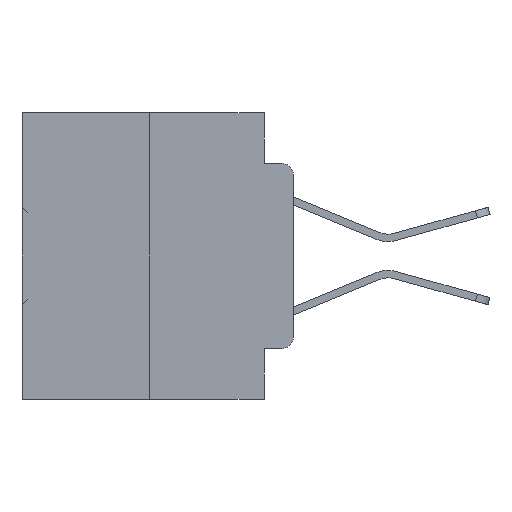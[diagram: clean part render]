
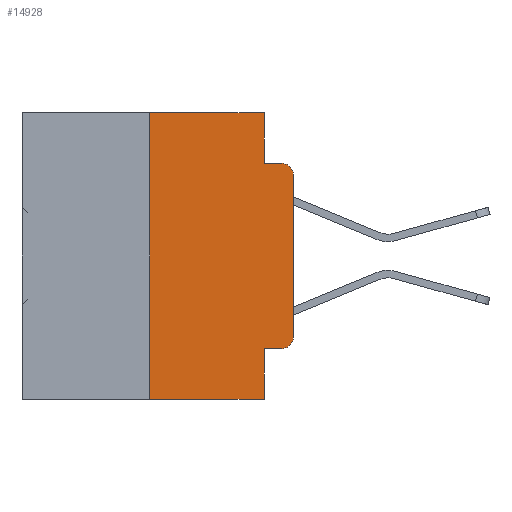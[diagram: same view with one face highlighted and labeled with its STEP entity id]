
A CAD part, left-side view. The second image highlights one B-rep face of the part: STEP entity #14928.
In plain terms, the highlighted planar face has unit normal (-1, 0, 0).
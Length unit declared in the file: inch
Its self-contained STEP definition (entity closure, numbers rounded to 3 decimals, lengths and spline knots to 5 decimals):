
#336 = AXIS2_PLACEMENT_3D ( 'NONE', #9981, #27452, #23867 ) ;
#346 = CARTESIAN_POINT ( 'NONE',  ( 0., 0.25, -0.5 ) ) ;
#2076 = LINE ( 'NONE', #24842, #9273 ) ;
#2469 = CARTESIAN_POINT ( 'NONE',  ( 0., 0.473, -0.5 ) ) ;
#2613 = VERTEX_POINT ( 'NONE', #22245 ) ;
#2767 = FACE_OUTER_BOUND ( 'NONE', #27448, .T. ) ;
#3425 = VERTEX_POINT ( 'NONE', #19836 ) ;
#4374 = CARTESIAN_POINT ( 'NONE',  ( 0., 0.25, 0. ) ) ;
#4481 = AXIS2_PLACEMENT_3D ( 'NONE', #8803, #14327, #31788 ) ;
#4560 = CARTESIAN_POINT ( 'NONE',  ( 0., 0., 0. ) ) ;
#4737 = CARTESIAN_POINT ( 'NONE',  ( 0., 0.051, -0.4115 ) ) ;
#4744 = LINE ( 'NONE', #4560, #4888 ) ;
#4888 = VECTOR ( 'NONE', #34183, 39.37008 ) ;
#5615 = DIRECTION ( 'NONE',  ( 1., 0., 0. ) ) ;
#7389 = VERTEX_POINT ( 'NONE', #4737 ) ;
#8803 = CARTESIAN_POINT ( 'NONE',  ( 0., 0.02, -0.3915 ) ) ;
#9038 = VERTEX_POINT ( 'NONE', #32621 ) ;
#9273 = VECTOR ( 'NONE', #10605, 39.37008 ) ;
#9511 = EDGE_CURVE ( 'NONE', #25197, #33193, #15458, .T. ) ;
#9569 = VERTEX_POINT ( 'NONE', #10919 ) ;
#9981 = CARTESIAN_POINT ( 'NONE',  ( 0., 0.02, -0.1085 ) ) ;
#10116 = ORIENTED_EDGE ( 'NONE', *, *, #35758, .F. ) ;
#10256 = CARTESIAN_POINT ( 'NONE',  ( 0., 0., -0.1085 ) ) ;
#10286 = VERTEX_POINT ( 'NONE', #19867 ) ;
#10605 = DIRECTION ( 'NONE',  ( 0., 0., -1. ) ) ;
#10919 = CARTESIAN_POINT ( 'NONE',  ( 0., 0.051, -0.5 ) ) ;
#10961 = DIRECTION ( 'NONE',  ( 0., -1., 0. ) ) ;
#11130 = PLANE ( 'NONE',  #31583 ) ;
#11311 = CARTESIAN_POINT ( 'NONE',  ( 0., 0.473, 0. ) ) ;
#12053 = CARTESIAN_POINT ( 'NONE',  ( 0., 0.02, -0.0885 ) ) ;
#12100 = DIRECTION ( 'NONE',  ( 0., 0., -1. ) ) ;
#14327 = DIRECTION ( 'NONE',  ( -1., 0., 0. ) ) ;
#14928 = ADVANCED_FACE ( 'NONE', ( #2767 ), #11130, .F. ) ;
#15067 = ORIENTED_EDGE ( 'NONE', *, *, #36585, .F. ) ;
#15159 = VECTOR ( 'NONE', #29651, 39.37008 ) ;
#15458 = CIRCLE ( 'NONE', #336, 0.02 ) ;
#15583 = CARTESIAN_POINT ( 'NONE',  ( 0., 0.473, 0. ) ) ;
#16803 = ORIENTED_EDGE ( 'NONE', *, *, #21472, .T. ) ;
#16809 = EDGE_CURVE ( 'NONE', #3425, #10286, #30028, .T. ) ;
#17097 = LINE ( 'NONE', #2469, #32312 ) ;
#19068 = VECTOR ( 'NONE', #10961, 39.37008 ) ;
#19418 = EDGE_CURVE ( 'NONE', #2613, #33244, #20881, .T. ) ;
#19578 = DIRECTION ( 'NONE',  ( 0., -1., 0. ) ) ;
#19836 = CARTESIAN_POINT ( 'NONE',  ( 0., 0.25, 0. ) ) ;
#19867 = CARTESIAN_POINT ( 'NONE',  ( 0., 0.051, 0. ) ) ;
#19955 = VECTOR ( 'NONE', #23955, 39.37008 ) ;
#20004 = LINE ( 'NONE', #22857, #29765 ) ;
#20559 = DIRECTION ( 'NONE',  ( 0., -1., 0. ) ) ;
#20881 = CIRCLE ( 'NONE', #4481, 0.02 ) ;
#21472 = EDGE_CURVE ( 'NONE', #33244, #25197, #4744, .T. ) ;
#21493 = ORIENTED_EDGE ( 'NONE', *, *, #9511, .T. ) ;
#22245 = CARTESIAN_POINT ( 'NONE',  ( 0., 0.02, -0.4115 ) ) ;
#22857 = CARTESIAN_POINT ( 'NONE',  ( 0., 0.051, -0.0885 ) ) ;
#23867 = DIRECTION ( 'NONE',  ( 0., 0., -1. ) ) ;
#23955 = DIRECTION ( 'NONE',  ( 0., 0., 1. ) ) ;
#24072 = ORIENTED_EDGE ( 'NONE', *, *, #25340, .T. ) ;
#24842 = CARTESIAN_POINT ( 'NONE',  ( 0., 0.051, 0. ) ) ;
#25197 = VERTEX_POINT ( 'NONE', #10256 ) ;
#25340 = EDGE_CURVE ( 'NONE', #36489, #9569, #17097, .T. ) ;
#26782 = EDGE_CURVE ( 'NONE', #7389, #2613, #30327, .T. ) ;
#26914 = CARTESIAN_POINT ( 'NONE',  ( 0., 0.051, 0. ) ) ;
#27169 = LINE ( 'NONE', #4374, #19955 ) ;
#27448 = EDGE_LOOP ( 'NONE', ( #16803, #21493, #28653, #34594, #31407, #10116, #24072, #15067, #30449, #33677 ) ) ;
#27452 = DIRECTION ( 'NONE',  ( -1., 0., 0. ) ) ;
#28653 = ORIENTED_EDGE ( 'NONE', *, *, #28815, .F. ) ;
#28815 = EDGE_CURVE ( 'NONE', #9038, #33193, #20004, .T. ) ;
#29651 = DIRECTION ( 'NONE',  ( 0., -1., 0. ) ) ;
#29765 = VECTOR ( 'NONE', #20559, 39.37008 ) ;
#30028 = LINE ( 'NONE', #15583, #15159 ) ;
#30072 = CARTESIAN_POINT ( 'NONE',  ( 0., 0., -0.3915 ) ) ;
#30317 = VECTOR ( 'NONE', #12100, 39.37008 ) ;
#30327 = LINE ( 'NONE', #33744, #19068 ) ;
#30449 = ORIENTED_EDGE ( 'NONE', *, *, #26782, .T. ) ;
#31407 = ORIENTED_EDGE ( 'NONE', *, *, #16809, .F. ) ;
#31583 = AXIS2_PLACEMENT_3D ( 'NONE', #11311, #5615, #34470 ) ;
#31788 = DIRECTION ( 'NONE',  ( 0., 0., -1. ) ) ;
#32312 = VECTOR ( 'NONE', #19578, 39.37008 ) ;
#32472 = EDGE_CURVE ( 'NONE', #10286, #9038, #2076, .T. ) ;
#32621 = CARTESIAN_POINT ( 'NONE',  ( 0., 0.051, -0.0885 ) ) ;
#32773 = LINE ( 'NONE', #26914, #30317 ) ;
#33193 = VERTEX_POINT ( 'NONE', #12053 ) ;
#33244 = VERTEX_POINT ( 'NONE', #30072 ) ;
#33677 = ORIENTED_EDGE ( 'NONE', *, *, #19418, .T. ) ;
#33744 = CARTESIAN_POINT ( 'NONE',  ( 0., 0.051, -0.4115 ) ) ;
#34183 = DIRECTION ( 'NONE',  ( 0., 0., 1. ) ) ;
#34470 = DIRECTION ( 'NONE',  ( 0., 0., -1. ) ) ;
#34594 = ORIENTED_EDGE ( 'NONE', *, *, #32472, .F. ) ;
#35758 = EDGE_CURVE ( 'NONE', #36489, #3425, #27169, .T. ) ;
#36489 = VERTEX_POINT ( 'NONE', #346 ) ;
#36585 = EDGE_CURVE ( 'NONE', #7389, #9569, #32773, .T. ) ;
